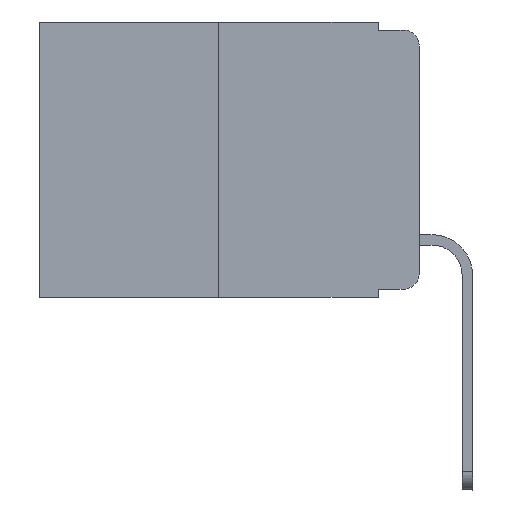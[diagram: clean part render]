
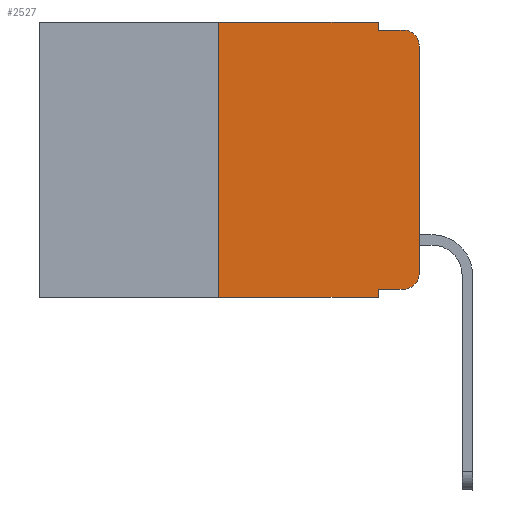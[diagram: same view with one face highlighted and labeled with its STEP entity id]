
A CAD part, left-side view. The second image highlights one B-rep face of the part: STEP entity #2527.
In plain terms, the highlighted planar face has unit normal (-1, 0, 0).
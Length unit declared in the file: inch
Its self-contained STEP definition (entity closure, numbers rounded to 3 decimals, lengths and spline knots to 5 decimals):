
#379 = VERTEX_POINT ( 'NONE', #7008 ) ;
#423 = VECTOR ( 'NONE', #3989, 39.37008 ) ;
#520 = DIRECTION ( 'NONE',  ( 1., 0., 0. ) ) ;
#739 = ORIENTED_EDGE ( 'NONE', *, *, #1651, .F. ) ;
#752 = VERTEX_POINT ( 'NONE', #2800 ) ;
#1281 = ORIENTED_EDGE ( 'NONE', *, *, #9351, .F. ) ;
#1348 = LINE ( 'NONE', #7269, #11120 ) ;
#1633 = ORIENTED_EDGE ( 'NONE', *, *, #6761, .T. ) ;
#1651 = EDGE_CURVE ( 'NONE', #2205, #379, #11874, .T. ) ;
#1679 = DIRECTION ( 'NONE',  ( 0., 0., -1. ) ) ;
#1705 = VERTEX_POINT ( 'NONE', #7012 ) ;
#1835 = CARTESIAN_POINT ( 'NONE',  ( 0., 0.051, -0.333 ) ) ;
#2205 = VERTEX_POINT ( 'NONE', #9068 ) ;
#2325 = DIRECTION ( 'NONE',  ( 0., 0., -1. ) ) ;
#2363 = ORIENTED_EDGE ( 'NONE', *, *, #5773, .T. ) ;
#2443 = CARTESIAN_POINT ( 'NONE',  ( 0., 0.051, 0. ) ) ;
#2527 = ADVANCED_FACE ( 'NONE', ( #5485 ), #8110, .F. ) ;
#2800 = CARTESIAN_POINT ( 'NONE',  ( 0., 0.051, 0. ) ) ;
#2878 = CARTESIAN_POINT ( 'NONE',  ( 0., 0.02, -0.03 ) ) ;
#3424 = DIRECTION ( 'NONE',  ( 0., 0., -1. ) ) ;
#3534 = VERTEX_POINT ( 'NONE', #10273 ) ;
#3989 = DIRECTION ( 'NONE',  ( 0., -1., 0. ) ) ;
#4081 = DIRECTION ( 'NONE',  ( 0., 0., -1. ) ) ;
#4144 = LINE ( 'NONE', #7053, #9017 ) ;
#4171 = DIRECTION ( 'NONE',  ( 0., 0., 1. ) ) ;
#4297 = CARTESIAN_POINT ( 'NONE',  ( 0., 0.25, 0. ) ) ;
#4311 = LINE ( 'NONE', #12264, #7905 ) ;
#4346 = AXIS2_PLACEMENT_3D ( 'NONE', #8286, #520, #3424 ) ;
#4845 = ORIENTED_EDGE ( 'NONE', *, *, #9474, .T. ) ;
#4913 = ORIENTED_EDGE ( 'NONE', *, *, #5095, .F. ) ;
#5024 = AXIS2_PLACEMENT_3D ( 'NONE', #12399, #6638, #1679 ) ;
#5095 = EDGE_CURVE ( 'NONE', #12378, #3534, #4144, .T. ) ;
#5148 = LINE ( 'NONE', #4297, #5549 ) ;
#5214 = EDGE_CURVE ( 'NONE', #11038, #3534, #10137, .T. ) ;
#5231 = CARTESIAN_POINT ( 'NONE',  ( 0., 0., 0. ) ) ;
#5307 = DIRECTION ( 'NONE',  ( 0., -1., 0. ) ) ;
#5420 = CIRCLE ( 'NONE', #5024, 0.02 ) ;
#5485 = FACE_OUTER_BOUND ( 'NONE', #8422, .T. ) ;
#5549 = VECTOR ( 'NONE', #4171, 39.37008 ) ;
#5556 = AXIS2_PLACEMENT_3D ( 'NONE', #2878, #6885, #8725 ) ;
#5601 = VECTOR ( 'NONE', #5307, 39.37008 ) ;
#5773 = EDGE_CURVE ( 'NONE', #5937, #6355, #5420, .T. ) ;
#5774 = ORIENTED_EDGE ( 'NONE', *, *, #9305, .T. ) ;
#5937 = VERTEX_POINT ( 'NONE', #9937 ) ;
#6026 = ORIENTED_EDGE ( 'NONE', *, *, #6932, .F. ) ;
#6355 = VERTEX_POINT ( 'NONE', #6812 ) ;
#6473 = VECTOR ( 'NONE', #8156, 39.37008 ) ;
#6638 = DIRECTION ( 'NONE',  ( -1., 0., 0. ) ) ;
#6702 = ORIENTED_EDGE ( 'NONE', *, *, #8947, .F. ) ;
#6761 = EDGE_CURVE ( 'NONE', #1705, #379, #9820, .T. ) ;
#6812 = CARTESIAN_POINT ( 'NONE',  ( 0., 0., -0.313 ) ) ;
#6885 = DIRECTION ( 'NONE',  ( -1., 0., 0. ) ) ;
#6886 = CARTESIAN_POINT ( 'NONE',  ( 0., 0.051, -0.01 ) ) ;
#6932 = EDGE_CURVE ( 'NONE', #11038, #8168, #5148, .T. ) ;
#7008 = CARTESIAN_POINT ( 'NONE',  ( 0., 0.02, -0.01 ) ) ;
#7012 = CARTESIAN_POINT ( 'NONE',  ( 0., 0., -0.03 ) ) ;
#7053 = CARTESIAN_POINT ( 'NONE',  ( 0., 0.051, 0. ) ) ;
#7228 = CARTESIAN_POINT ( 'NONE',  ( 0., 0.473, -0.343 ) ) ;
#7269 = CARTESIAN_POINT ( 'NONE',  ( 0., 0.051, -0.333 ) ) ;
#7470 = LINE ( 'NONE', #2443, #7894 ) ;
#7894 = VECTOR ( 'NONE', #2325, 39.37008 ) ;
#7905 = VECTOR ( 'NONE', #9291, 39.37008 ) ;
#8110 = PLANE ( 'NONE',  #4346 ) ;
#8156 = DIRECTION ( 'NONE',  ( 0., 0., 1. ) ) ;
#8168 = VERTEX_POINT ( 'NONE', #9088 ) ;
#8286 = CARTESIAN_POINT ( 'NONE',  ( 0., 0.473, 0. ) ) ;
#8400 = LINE ( 'NONE', #5231, #6473 ) ;
#8422 = EDGE_LOOP ( 'NONE', ( #5774, #1633, #739, #6702, #1281, #6026, #12532, #4913, #4845, #2363 ) ) ;
#8570 = CARTESIAN_POINT ( 'NONE',  ( 0., 0.25, -0.343 ) ) ;
#8725 = DIRECTION ( 'NONE',  ( 0., 0., -1. ) ) ;
#8947 = EDGE_CURVE ( 'NONE', #752, #2205, #7470, .T. ) ;
#9017 = VECTOR ( 'NONE', #4081, 39.37008 ) ;
#9068 = CARTESIAN_POINT ( 'NONE',  ( 0., 0.051, -0.01 ) ) ;
#9088 = CARTESIAN_POINT ( 'NONE',  ( 0., 0.25, 0. ) ) ;
#9291 = DIRECTION ( 'NONE',  ( 0., -1., 0. ) ) ;
#9305 = EDGE_CURVE ( 'NONE', #6355, #1705, #8400, .T. ) ;
#9351 = EDGE_CURVE ( 'NONE', #8168, #752, #4311, .T. ) ;
#9474 = EDGE_CURVE ( 'NONE', #12378, #5937, #1348, .T. ) ;
#9820 = CIRCLE ( 'NONE', #5556, 0.02 ) ;
#9937 = CARTESIAN_POINT ( 'NONE',  ( 0., 0.02, -0.333 ) ) ;
#10137 = LINE ( 'NONE', #7228, #5601 ) ;
#10172 = DIRECTION ( 'NONE',  ( 0., -1., 0. ) ) ;
#10273 = CARTESIAN_POINT ( 'NONE',  ( 0., 0.051, -0.343 ) ) ;
#11038 = VERTEX_POINT ( 'NONE', #8570 ) ;
#11120 = VECTOR ( 'NONE', #10172, 39.37008 ) ;
#11874 = LINE ( 'NONE', #6886, #423 ) ;
#12264 = CARTESIAN_POINT ( 'NONE',  ( 0., 0.473, 0. ) ) ;
#12378 = VERTEX_POINT ( 'NONE', #1835 ) ;
#12399 = CARTESIAN_POINT ( 'NONE',  ( 0., 0.02, -0.313 ) ) ;
#12532 = ORIENTED_EDGE ( 'NONE', *, *, #5214, .T. ) ;
